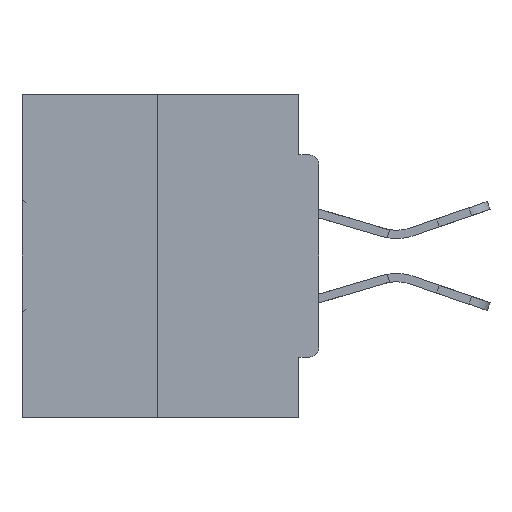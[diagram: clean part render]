
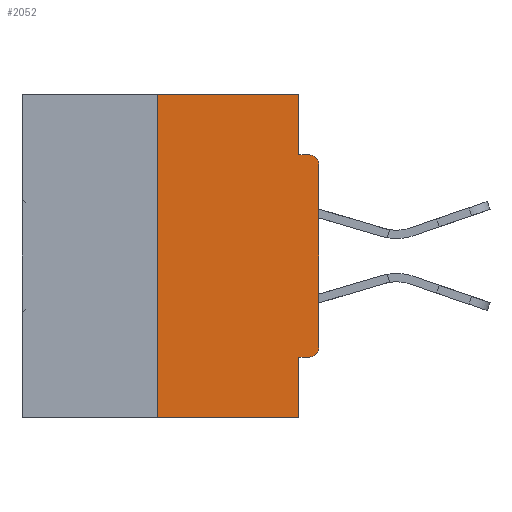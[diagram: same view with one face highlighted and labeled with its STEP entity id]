
A CAD part, left-side view. The second image highlights one B-rep face of the part: STEP entity #2052.
In plain terms, the highlighted planar face has unit normal (-1, 0, 0).
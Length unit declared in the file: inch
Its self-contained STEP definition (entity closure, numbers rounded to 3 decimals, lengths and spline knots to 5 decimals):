
#43 = ORIENTED_EDGE ( 'NONE', *, *, #2164, .F. ) ;
#214 = ORIENTED_EDGE ( 'NONE', *, *, #9691, .T. ) ;
#353 = DIRECTION ( 'NONE',  ( 0., 0., 1. ) ) ;
#468 = VECTOR ( 'NONE', #43271, 39.37008 ) ;
#1038 = DIRECTION ( 'NONE',  ( 0., 1., 0. ) ) ;
#1228 = DIRECTION ( 'NONE',  ( 0., 0., -1. ) ) ;
#1316 = AXIS2_PLACEMENT_3D ( 'NONE', #20753, #3760, #42145 ) ;
#1577 = ORIENTED_EDGE ( 'NONE', *, *, #4504, .T. ) ;
#2052 = ADVANCED_FACE ( 'NONE', ( #36052 ), #17401, .F. ) ;
#2164 = EDGE_CURVE ( 'NONE', #26575, #7507, #18655, .T. ) ;
#2482 = DIRECTION ( 'NONE',  ( -1., 0., 0. ) ) ;
#2589 = ORIENTED_EDGE ( 'NONE', *, *, #13754, .F. ) ;
#2802 = CARTESIAN_POINT ( 'NONE',  ( 0., 0.46, -0.5 ) ) ;
#3760 = DIRECTION ( 'NONE',  ( 1., 0., 0. ) ) ;
#4504 = EDGE_CURVE ( 'NONE', #26575, #14267, #16272, .T. ) ;
#4726 = VERTEX_POINT ( 'NONE', #26994 ) ;
#4817 = ORIENTED_EDGE ( 'NONE', *, *, #4905, .T. ) ;
#4905 = EDGE_CURVE ( 'NONE', #4726, #39985, #42810, .T. ) ;
#6568 = CARTESIAN_POINT ( 'NONE',  ( 0., 0.015, -0.0935 ) ) ;
#6671 = CARTESIAN_POINT ( 'NONE',  ( 0., 0., -0.3915 ) ) ;
#7507 = VERTEX_POINT ( 'NONE', #17134 ) ;
#8734 = DIRECTION ( 'NONE',  ( 0., 0., -1. ) ) ;
#9691 = EDGE_CURVE ( 'NONE', #14267, #17058, #35129, .T. ) ;
#10003 = DIRECTION ( 'NONE',  ( 0., 0., 1. ) ) ;
#10075 = VECTOR ( 'NONE', #8734, 39.37008 ) ;
#10587 = VERTEX_POINT ( 'NONE', #6568 ) ;
#13754 = EDGE_CURVE ( 'NONE', #24710, #10587, #26446, .T. ) ;
#13978 = ORIENTED_EDGE ( 'NONE', *, *, #24988, .F. ) ;
#14267 = VERTEX_POINT ( 'NONE', #6671 ) ;
#14278 = CARTESIAN_POINT ( 'NONE',  ( 0., 0., 0. ) ) ;
#16231 = VECTOR ( 'NONE', #30742, 39.37008 ) ;
#16272 = CIRCLE ( 'NONE', #33248, 0.015 ) ;
#17058 = VERTEX_POINT ( 'NONE', #36005 ) ;
#17134 = CARTESIAN_POINT ( 'NONE',  ( 0., 0.031, -0.4065 ) ) ;
#17191 = VECTOR ( 'NONE', #44981, 39.37008 ) ;
#17401 = PLANE ( 'NONE',  #1316 ) ;
#18404 = CARTESIAN_POINT ( 'NONE',  ( 0., 0.031, 0. ) ) ;
#18655 = LINE ( 'NONE', #38808, #30080 ) ;
#20678 = CARTESIAN_POINT ( 'NONE',  ( 0., 0., -0.0935 ) ) ;
#20753 = CARTESIAN_POINT ( 'NONE',  ( 0., 0.46, 0. ) ) ;
#22138 = CARTESIAN_POINT ( 'NONE',  ( 0., 0.015, -0.3915 ) ) ;
#22787 = CARTESIAN_POINT ( 'NONE',  ( 0., 0.015, -0.4065 ) ) ;
#23030 = CARTESIAN_POINT ( 'NONE',  ( 0., 0.031, -0.5 ) ) ;
#23610 = AXIS2_PLACEMENT_3D ( 'NONE', #37232, #2482, #33899 ) ;
#23635 = CARTESIAN_POINT ( 'NONE',  ( 0., 0.031, -0.5 ) ) ;
#23878 = CARTESIAN_POINT ( 'NONE',  ( 0., 0.25, 0. ) ) ;
#24057 = EDGE_CURVE ( 'NONE', #26602, #24710, #42926, .T. ) ;
#24123 = ORIENTED_EDGE ( 'NONE', *, *, #33707, .F. ) ;
#24710 = VERTEX_POINT ( 'NONE', #25191 ) ;
#24988 = EDGE_CURVE ( 'NONE', #7507, #39985, #44893, .T. ) ;
#25191 = CARTESIAN_POINT ( 'NONE',  ( 0., 0.031, -0.0935 ) ) ;
#25247 = EDGE_LOOP ( 'NONE', ( #42302, #24123, #4817, #13978, #43, #1577, #214, #33263, #2589, #38841 ) ) ;
#26446 = LINE ( 'NONE', #20678, #17191 ) ;
#26575 = VERTEX_POINT ( 'NONE', #22787 ) ;
#26602 = VERTEX_POINT ( 'NONE', #32718 ) ;
#26994 = CARTESIAN_POINT ( 'NONE',  ( 0., 0.25, -0.5 ) ) ;
#28851 = DIRECTION ( 'NONE',  ( -1., 0., 0. ) ) ;
#29162 = VECTOR ( 'NONE', #353, 39.37008 ) ;
#29693 = DIRECTION ( 'NONE',  ( 0., -1., 0. ) ) ;
#30080 = VECTOR ( 'NONE', #1038, 39.37008 ) ;
#30100 = VECTOR ( 'NONE', #10003, 39.37008 ) ;
#30742 = DIRECTION ( 'NONE',  ( 0., -1., 0. ) ) ;
#32718 = CARTESIAN_POINT ( 'NONE',  ( 0., 0.031, 0. ) ) ;
#32740 = CARTESIAN_POINT ( 'NONE',  ( 0., 0.46, 0. ) ) ;
#33248 = AXIS2_PLACEMENT_3D ( 'NONE', #22138, #28851, #1228 ) ;
#33263 = ORIENTED_EDGE ( 'NONE', *, *, #41443, .T. ) ;
#33707 = EDGE_CURVE ( 'NONE', #4726, #40557, #39312, .T. ) ;
#33899 = DIRECTION ( 'NONE',  ( 0., 0., -1. ) ) ;
#35129 = LINE ( 'NONE', #14278, #29162 ) ;
#35722 = CARTESIAN_POINT ( 'NONE',  ( 0., 0.25, 0. ) ) ;
#36005 = CARTESIAN_POINT ( 'NONE',  ( 0., 0., -0.1085 ) ) ;
#36052 = FACE_OUTER_BOUND ( 'NONE', #25247, .T. ) ;
#36504 = EDGE_CURVE ( 'NONE', #40557, #26602, #43461, .T. ) ;
#37232 = CARTESIAN_POINT ( 'NONE',  ( 0., 0.015, -0.1085 ) ) ;
#37496 = VECTOR ( 'NONE', #29693, 39.37008 ) ;
#38808 = CARTESIAN_POINT ( 'NONE',  ( 0., 0., -0.4065 ) ) ;
#38841 = ORIENTED_EDGE ( 'NONE', *, *, #24057, .F. ) ;
#39312 = LINE ( 'NONE', #23878, #30100 ) ;
#39985 = VERTEX_POINT ( 'NONE', #23635 ) ;
#40557 = VERTEX_POINT ( 'NONE', #35722 ) ;
#41226 = CIRCLE ( 'NONE', #23610, 0.015 ) ;
#41443 = EDGE_CURVE ( 'NONE', #17058, #10587, #41226, .T. ) ;
#42145 = DIRECTION ( 'NONE',  ( 0., 0., -1. ) ) ;
#42302 = ORIENTED_EDGE ( 'NONE', *, *, #36504, .F. ) ;
#42810 = LINE ( 'NONE', #2802, #16231 ) ;
#42926 = LINE ( 'NONE', #18404, #468 ) ;
#43271 = DIRECTION ( 'NONE',  ( 0., 0., -1. ) ) ;
#43461 = LINE ( 'NONE', #32740, #37496 ) ;
#44893 = LINE ( 'NONE', #23030, #10075 ) ;
#44981 = DIRECTION ( 'NONE',  ( 0., -1., 0. ) ) ;
